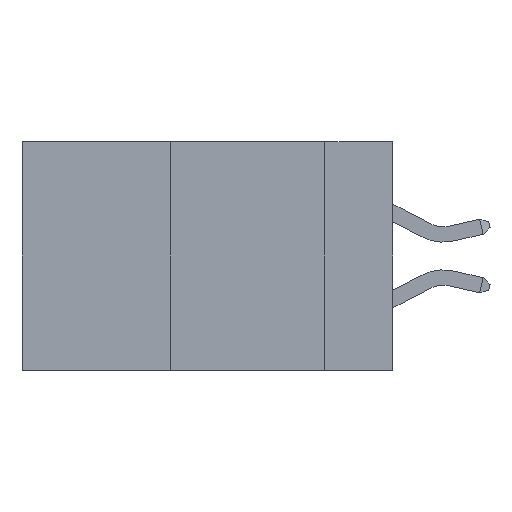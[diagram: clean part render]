
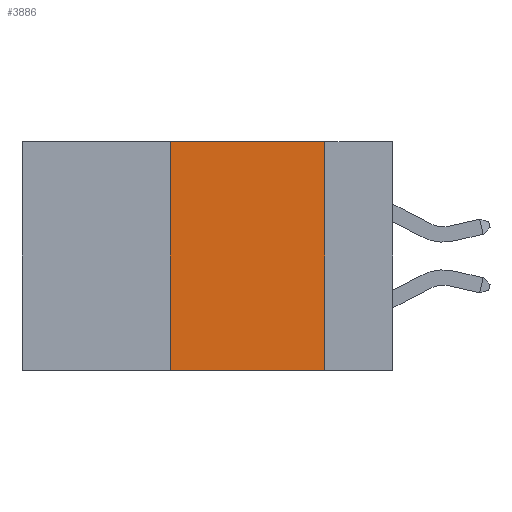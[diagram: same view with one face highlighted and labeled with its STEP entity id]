
A CAD part, left-side view. The second image highlights one B-rep face of the part: STEP entity #3886.
In plain terms, the highlighted planar face has unit normal (-1, 0, 0).
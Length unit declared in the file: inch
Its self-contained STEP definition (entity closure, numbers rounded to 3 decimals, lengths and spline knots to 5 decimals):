
#2 = LINE ( 'NONE', #9618, #12780 ) ;
#3 = ORIENTED_EDGE ( 'NONE', *, *, #3877, .F. ) ;
#12 = VERTEX_POINT ( 'NONE', #10731 ) ;
#475 = VERTEX_POINT ( 'NONE', #12293 ) ;
#811 = DIRECTION ( 'NONE',  ( 0., -1., 0. ) ) ;
#941 = ORIENTED_EDGE ( 'NONE', *, *, #12223, .T. ) ;
#1574 = CARTESIAN_POINT ( 'NONE',  ( 0., 0.11, -0.37 ) ) ;
#2519 = ORIENTED_EDGE ( 'NONE', *, *, #4535, .F. ) ;
#2742 = EDGE_LOOP ( 'NONE', ( #8808, #2519, #3, #941 ) ) ;
#2903 = VECTOR ( 'NONE', #10259, 39.37008 ) ;
#3525 = LINE ( 'NONE', #10866, #7311 ) ;
#3877 = EDGE_CURVE ( 'NONE', #475, #14269, #3525, .T. ) ;
#3886 = ADVANCED_FACE ( 'NONE', ( #6498 ), #12170, .F. ) ;
#4535 = EDGE_CURVE ( 'NONE', #14269, #12, #12678, .T. ) ;
#6182 = VECTOR ( 'NONE', #811, 39.37008 ) ;
#6498 = FACE_OUTER_BOUND ( 'NONE', #2742, .T. ) ;
#7037 = EDGE_CURVE ( 'NONE', #12, #9507, #2, .T. ) ;
#7311 = VECTOR ( 'NONE', #11901, 39.37008 ) ;
#8808 = ORIENTED_EDGE ( 'NONE', *, *, #7037, .F. ) ;
#9507 = VERTEX_POINT ( 'NONE', #1574 ) ;
#9618 = CARTESIAN_POINT ( 'NONE',  ( 0., 0.11, 0. ) ) ;
#9787 = LINE ( 'NONE', #13187, #6182 ) ;
#10041 = CARTESIAN_POINT ( 'NONE',  ( 0., 0.36, 0. ) ) ;
#10259 = DIRECTION ( 'NONE',  ( 0., -1., 0. ) ) ;
#10731 = CARTESIAN_POINT ( 'NONE',  ( 0., 0.11, 0. ) ) ;
#10866 = CARTESIAN_POINT ( 'NONE',  ( 0., 0.36, 0. ) ) ;
#11181 = DIRECTION ( 'NONE',  ( 0., 0., -1. ) ) ;
#11564 = DIRECTION ( 'NONE',  ( 1., 0., 0. ) ) ;
#11620 = CARTESIAN_POINT ( 'NONE',  ( 0., 0.6, 0. ) ) ;
#11901 = DIRECTION ( 'NONE',  ( 0., 0., 1. ) ) ;
#12170 = PLANE ( 'NONE',  #12902 ) ;
#12223 = EDGE_CURVE ( 'NONE', #475, #9507, #9787, .T. ) ;
#12293 = CARTESIAN_POINT ( 'NONE',  ( 0., 0.36, -0.37 ) ) ;
#12678 = LINE ( 'NONE', #11620, #2903 ) ;
#12780 = VECTOR ( 'NONE', #14295, 39.37008 ) ;
#12902 = AXIS2_PLACEMENT_3D ( 'NONE', #13001, #11564, #11181 ) ;
#13001 = CARTESIAN_POINT ( 'NONE',  ( 0., 0.6, 0. ) ) ;
#13187 = CARTESIAN_POINT ( 'NONE',  ( 0., 0.6, -0.37 ) ) ;
#14269 = VERTEX_POINT ( 'NONE', #10041 ) ;
#14295 = DIRECTION ( 'NONE',  ( 0., 0., -1. ) ) ;
